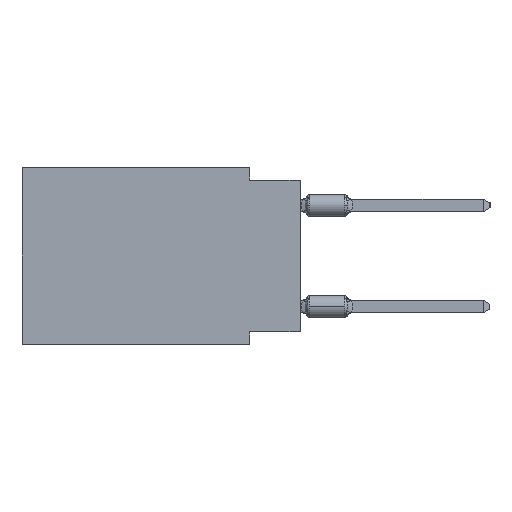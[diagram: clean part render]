
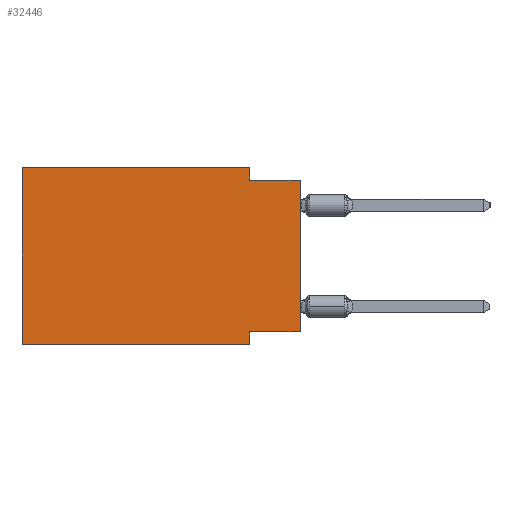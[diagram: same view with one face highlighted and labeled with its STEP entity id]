
A CAD part, left-side view. The second image highlights one B-rep face of the part: STEP entity #32446.
In plain terms, the highlighted planar face has unit normal (-1, 0, 0).
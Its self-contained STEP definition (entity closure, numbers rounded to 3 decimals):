
#370 = ORIENTED_EDGE ( 'NONE', *, *, #33378, .F. ) ;
#911 = LINE ( 'NONE', #28106, #16016 ) ;
#1301 = CARTESIAN_POINT ( 'NONE',  ( 0., 2.54, -8.89 ) ) ;
#2006 = CARTESIAN_POINT ( 'NONE',  ( 0., 13.97, -8.89 ) ) ;
#2235 = CARTESIAN_POINT ( 'NONE',  ( 0., 2.54, 0. ) ) ;
#2518 = LINE ( 'NONE', #27208, #26064 ) ;
#4031 = AXIS2_PLACEMENT_3D ( 'NONE', #11414, #7610, #31635 ) ;
#4966 = DIRECTION ( 'NONE',  ( 0., 0., 1. ) ) ;
#5516 = VECTOR ( 'NONE', #41135, 1000. ) ;
#5811 = LINE ( 'NONE', #2006, #16411 ) ;
#5938 = EDGE_CURVE ( 'NONE', #6060, #27323, #13266, .T. ) ;
#6060 = VERTEX_POINT ( 'NONE', #24657 ) ;
#6234 = CARTESIAN_POINT ( 'NONE',  ( 0., 2.54, -8.255 ) ) ;
#7610 = DIRECTION ( 'NONE',  ( 1., 0., 0. ) ) ;
#8998 = CARTESIAN_POINT ( 'NONE',  ( 0., 13.97, 0. ) ) ;
#10381 = LINE ( 'NONE', #13973, #32837 ) ;
#11414 = CARTESIAN_POINT ( 'NONE',  ( 0., 13.97, 0. ) ) ;
#13266 = LINE ( 'NONE', #33506, #15028 ) ;
#13392 = VERTEX_POINT ( 'NONE', #18798 ) ;
#13496 = CARTESIAN_POINT ( 'NONE',  ( 0., 0., -8.255 ) ) ;
#13973 = CARTESIAN_POINT ( 'NONE',  ( 0., 0., -8.255 ) ) ;
#14615 = DIRECTION ( 'NONE',  ( 0., -1., 0. ) ) ;
#15028 = VECTOR ( 'NONE', #16635, 1000. ) ;
#15921 = DIRECTION ( 'NONE',  ( 0., 0., -1. ) ) ;
#16016 = VECTOR ( 'NONE', #14615, 1000. ) ;
#16211 = CARTESIAN_POINT ( 'NONE',  ( 0., 2.54, -0.635 ) ) ;
#16411 = VECTOR ( 'NONE', #26702, 1000. ) ;
#16635 = DIRECTION ( 'NONE',  ( 0., -1., 0. ) ) ;
#16784 = VECTOR ( 'NONE', #15921, 1000. ) ;
#18260 = VERTEX_POINT ( 'NONE', #1301 ) ;
#18320 = ORIENTED_EDGE ( 'NONE', *, *, #32105, .F. ) ;
#18640 = ORIENTED_EDGE ( 'NONE', *, *, #36754, .T. ) ;
#18798 = CARTESIAN_POINT ( 'NONE',  ( 0., 0., -0.635 ) ) ;
#19362 = EDGE_LOOP ( 'NONE', ( #39686, #31037, #20906, #34663, #18320, #18640, #370, #28912 ) ) ;
#19615 = VERTEX_POINT ( 'NONE', #6234 ) ;
#20906 = ORIENTED_EDGE ( 'NONE', *, *, #41625, .F. ) ;
#21160 = LINE ( 'NONE', #34188, #5516 ) ;
#21228 = VERTEX_POINT ( 'NONE', #16211 ) ;
#22902 = VERTEX_POINT ( 'NONE', #13496 ) ;
#24657 = CARTESIAN_POINT ( 'NONE',  ( 0., 13.97, 0. ) ) ;
#26064 = VECTOR ( 'NONE', #26551, 1000. ) ;
#26551 = DIRECTION ( 'NONE',  ( 0., 0., 1. ) ) ;
#26702 = DIRECTION ( 'NONE',  ( 0., -1., 0. ) ) ;
#27208 = CARTESIAN_POINT ( 'NONE',  ( 0., 0., 0. ) ) ;
#27323 = VERTEX_POINT ( 'NONE', #29866 ) ;
#28106 = CARTESIAN_POINT ( 'NONE',  ( 0., 0., -0.635 ) ) ;
#28398 = VECTOR ( 'NONE', #4966, 1000. ) ;
#28912 = ORIENTED_EDGE ( 'NONE', *, *, #35972, .F. ) ;
#29686 = CARTESIAN_POINT ( 'NONE',  ( 0., 13.97, -8.89 ) ) ;
#29866 = CARTESIAN_POINT ( 'NONE',  ( 0., 2.54, 0. ) ) ;
#31037 = ORIENTED_EDGE ( 'NONE', *, *, #31975, .F. ) ;
#31265 = DIRECTION ( 'NONE',  ( 0., 1., 0. ) ) ;
#31635 = DIRECTION ( 'NONE',  ( 0., 0., -1. ) ) ;
#31975 = EDGE_CURVE ( 'NONE', #21228, #13392, #911, .T. ) ;
#32105 = EDGE_CURVE ( 'NONE', #41175, #6060, #39767, .T. ) ;
#32446 = ADVANCED_FACE ( 'NONE', ( #35237 ), #38381, .F. ) ;
#32837 = VECTOR ( 'NONE', #31265, 1000. ) ;
#33378 = EDGE_CURVE ( 'NONE', #19615, #18260, #21160, .T. ) ;
#33506 = CARTESIAN_POINT ( 'NONE',  ( 0., 13.97, 0. ) ) ;
#34188 = CARTESIAN_POINT ( 'NONE',  ( 0., 2.54, -8.89 ) ) ;
#34663 = ORIENTED_EDGE ( 'NONE', *, *, #5938, .F. ) ;
#35237 = FACE_OUTER_BOUND ( 'NONE', #19362, .T. ) ;
#35972 = EDGE_CURVE ( 'NONE', #22902, #19615, #10381, .T. ) ;
#36593 = LINE ( 'NONE', #2235, #16784 ) ;
#36754 = EDGE_CURVE ( 'NONE', #41175, #18260, #5811, .T. ) ;
#38381 = PLANE ( 'NONE',  #4031 ) ;
#39686 = ORIENTED_EDGE ( 'NONE', *, *, #42421, .T. ) ;
#39767 = LINE ( 'NONE', #8998, #28398 ) ;
#41135 = DIRECTION ( 'NONE',  ( 0., 0., -1. ) ) ;
#41175 = VERTEX_POINT ( 'NONE', #29686 ) ;
#41625 = EDGE_CURVE ( 'NONE', #27323, #21228, #36593, .T. ) ;
#42421 = EDGE_CURVE ( 'NONE', #22902, #13392, #2518, .T. ) ;
